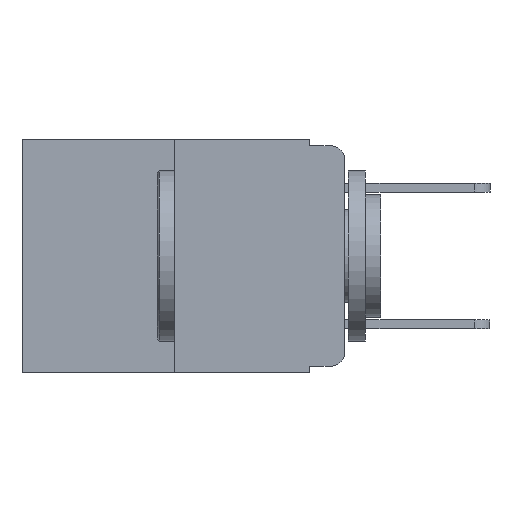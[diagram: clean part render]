
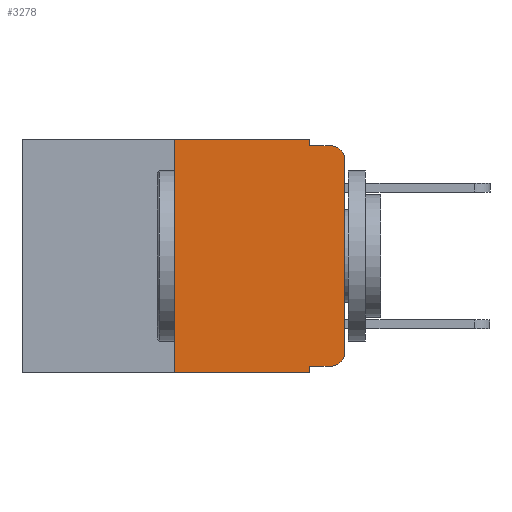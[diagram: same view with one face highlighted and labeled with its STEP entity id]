
A CAD part, left-side view. The second image highlights one B-rep face of the part: STEP entity #3278.
In plain terms, the highlighted planar face has unit normal (-1, 0, 0).
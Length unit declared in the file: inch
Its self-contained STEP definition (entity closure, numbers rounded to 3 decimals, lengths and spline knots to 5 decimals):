
#427 = ORIENTED_EDGE ( 'NONE', *, *, #6916, .F. ) ;
#533 = DIRECTION ( 'NONE',  ( -1., 0., 0. ) ) ;
#561 = ORIENTED_EDGE ( 'NONE', *, *, #9162, .T. ) ;
#588 = VECTOR ( 'NONE', #10586, 39.37008 ) ;
#774 = ORIENTED_EDGE ( 'NONE', *, *, #4099, .F. ) ;
#976 = LINE ( 'NONE', #2710, #9960 ) ;
#1014 = EDGE_CURVE ( 'NONE', #1857, #7211, #6985, .T. ) ;
#1111 = ORIENTED_EDGE ( 'NONE', *, *, #9971, .T. ) ;
#1121 = VECTOR ( 'NONE', #5485, 39.37008 ) ;
#1216 = CARTESIAN_POINT ( 'NONE',  ( 0., 0.051, 0. ) ) ;
#1288 = EDGE_CURVE ( 'NONE', #2623, #2118, #976, .T. ) ;
#1360 = CARTESIAN_POINT ( 'NONE',  ( 0., 0.051, 0. ) ) ;
#1482 = CARTESIAN_POINT ( 'NONE',  ( 0., 0.051, -0.333 ) ) ;
#1636 = DIRECTION ( 'NONE',  ( -1., 0., 0. ) ) ;
#1849 = VECTOR ( 'NONE', #8377, 39.37008 ) ;
#1857 = VERTEX_POINT ( 'NONE', #9984 ) ;
#1886 = EDGE_CURVE ( 'NONE', #5941, #2627, #4669, .T. ) ;
#2118 = VERTEX_POINT ( 'NONE', #8726 ) ;
#2175 = LINE ( 'NONE', #10265, #10806 ) ;
#2331 = DIRECTION ( 'NONE',  ( 0., 0., -1. ) ) ;
#2623 = VERTEX_POINT ( 'NONE', #1482 ) ;
#2627 = VERTEX_POINT ( 'NONE', #1360 ) ;
#2637 = VERTEX_POINT ( 'NONE', #4743 ) ;
#2667 = CARTESIAN_POINT ( 'NONE',  ( 0., 0., -0.03 ) ) ;
#2710 = CARTESIAN_POINT ( 'NONE',  ( 0., 0.051, -0.333 ) ) ;
#2735 = DIRECTION ( 'NONE',  ( 0., -1., 0. ) ) ;
#3193 = DIRECTION ( 'NONE',  ( 0., 0., -1. ) ) ;
#3278 = ADVANCED_FACE ( 'NONE', ( #10599 ), #8925, .F. ) ;
#3299 = CARTESIAN_POINT ( 'NONE',  ( 0., 0.051, -0.01 ) ) ;
#3583 = VERTEX_POINT ( 'NONE', #10448 ) ;
#3922 = LINE ( 'NONE', #1216, #9798 ) ;
#3934 = LINE ( 'NONE', #7831, #1121 ) ;
#4099 = EDGE_CURVE ( 'NONE', #2623, #2637, #5613, .T. ) ;
#4161 = CARTESIAN_POINT ( 'NONE',  ( 0., 0.02, -0.01 ) ) ;
#4195 = CARTESIAN_POINT ( 'NONE',  ( 0., 0.473, 0. ) ) ;
#4667 = CIRCLE ( 'NONE', #9100, 0.02 ) ;
#4669 = LINE ( 'NONE', #4195, #10176 ) ;
#4743 = CARTESIAN_POINT ( 'NONE',  ( 0., 0.051, -0.343 ) ) ;
#5122 = ORIENTED_EDGE ( 'NONE', *, *, #1288, .T. ) ;
#5194 = ORIENTED_EDGE ( 'NONE', *, *, #5764, .T. ) ;
#5239 = AXIS2_PLACEMENT_3D ( 'NONE', #8620, #8916, #3193 ) ;
#5485 = DIRECTION ( 'NONE',  ( 0., 0., 1. ) ) ;
#5613 = LINE ( 'NONE', #9403, #9279 ) ;
#5764 = EDGE_CURVE ( 'NONE', #3583, #2637, #2175, .T. ) ;
#5941 = VERTEX_POINT ( 'NONE', #11218 ) ;
#6150 = DIRECTION ( 'NONE',  ( 0., 0., -1. ) ) ;
#6289 = CARTESIAN_POINT ( 'NONE',  ( 0., 0.02, -0.03 ) ) ;
#6351 = EDGE_CURVE ( 'NONE', #3583, #5941, #3934, .T. ) ;
#6916 = EDGE_CURVE ( 'NONE', #2627, #8697, #3922, .T. ) ;
#6985 = LINE ( 'NONE', #8208, #1849 ) ;
#6998 = DIRECTION ( 'NONE',  ( 0., -1., 0. ) ) ;
#7064 = ORIENTED_EDGE ( 'NONE', *, *, #1886, .F. ) ;
#7095 = DIRECTION ( 'NONE',  ( 0., 0., -1. ) ) ;
#7107 = CARTESIAN_POINT ( 'NONE',  ( 0., 0.02, -0.313 ) ) ;
#7211 = VERTEX_POINT ( 'NONE', #2667 ) ;
#7226 = AXIS2_PLACEMENT_3D ( 'NONE', #7107, #1636, #7883 ) ;
#7831 = CARTESIAN_POINT ( 'NONE',  ( 0., 0.25, 0. ) ) ;
#7883 = DIRECTION ( 'NONE',  ( 0., 0., -1. ) ) ;
#7936 = EDGE_CURVE ( 'NONE', #8697, #10362, #9918, .T. ) ;
#8208 = CARTESIAN_POINT ( 'NONE',  ( 0., 0., 0. ) ) ;
#8377 = DIRECTION ( 'NONE',  ( 0., 0., 1. ) ) ;
#8620 = CARTESIAN_POINT ( 'NONE',  ( 0., 0.473, 0. ) ) ;
#8697 = VERTEX_POINT ( 'NONE', #9696 ) ;
#8726 = CARTESIAN_POINT ( 'NONE',  ( 0., 0.02, -0.333 ) ) ;
#8916 = DIRECTION ( 'NONE',  ( 1., 0., 0. ) ) ;
#8925 = PLANE ( 'NONE',  #5239 ) ;
#9023 = CIRCLE ( 'NONE', #7226, 0.02 ) ;
#9080 = EDGE_LOOP ( 'NONE', ( #10053, #1111, #10043, #427, #7064, #9118, #5194, #774, #5122, #561 ) ) ;
#9100 = AXIS2_PLACEMENT_3D ( 'NONE', #6289, #533, #7095 ) ;
#9118 = ORIENTED_EDGE ( 'NONE', *, *, #6351, .F. ) ;
#9162 = EDGE_CURVE ( 'NONE', #2118, #1857, #9023, .T. ) ;
#9279 = VECTOR ( 'NONE', #6150, 39.37008 ) ;
#9403 = CARTESIAN_POINT ( 'NONE',  ( 0., 0.051, 0. ) ) ;
#9551 = DIRECTION ( 'NONE',  ( 0., -1., 0. ) ) ;
#9696 = CARTESIAN_POINT ( 'NONE',  ( 0., 0.051, -0.01 ) ) ;
#9798 = VECTOR ( 'NONE', #2331, 39.37008 ) ;
#9918 = LINE ( 'NONE', #3299, #588 ) ;
#9960 = VECTOR ( 'NONE', #2735, 39.37008 ) ;
#9971 = EDGE_CURVE ( 'NONE', #7211, #10362, #4667, .T. ) ;
#9984 = CARTESIAN_POINT ( 'NONE',  ( 0., 0., -0.313 ) ) ;
#10043 = ORIENTED_EDGE ( 'NONE', *, *, #7936, .F. ) ;
#10053 = ORIENTED_EDGE ( 'NONE', *, *, #1014, .T. ) ;
#10176 = VECTOR ( 'NONE', #6998, 39.37008 ) ;
#10265 = CARTESIAN_POINT ( 'NONE',  ( 0., 0.473, -0.343 ) ) ;
#10362 = VERTEX_POINT ( 'NONE', #4161 ) ;
#10448 = CARTESIAN_POINT ( 'NONE',  ( 0., 0.25, -0.343 ) ) ;
#10586 = DIRECTION ( 'NONE',  ( 0., -1., 0. ) ) ;
#10599 = FACE_OUTER_BOUND ( 'NONE', #9080, .T. ) ;
#10806 = VECTOR ( 'NONE', #9551, 39.37008 ) ;
#11218 = CARTESIAN_POINT ( 'NONE',  ( 0., 0.25, 0. ) ) ;
